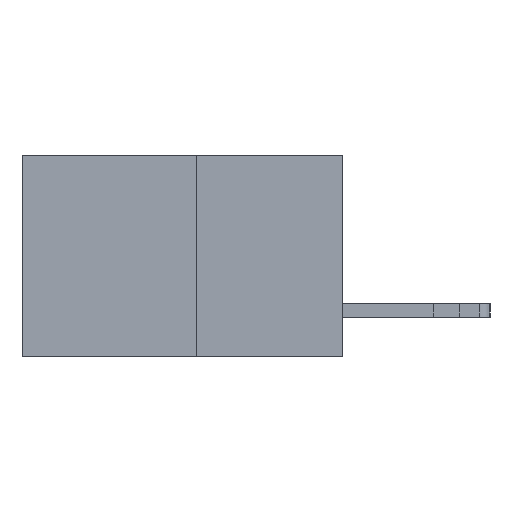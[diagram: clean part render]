
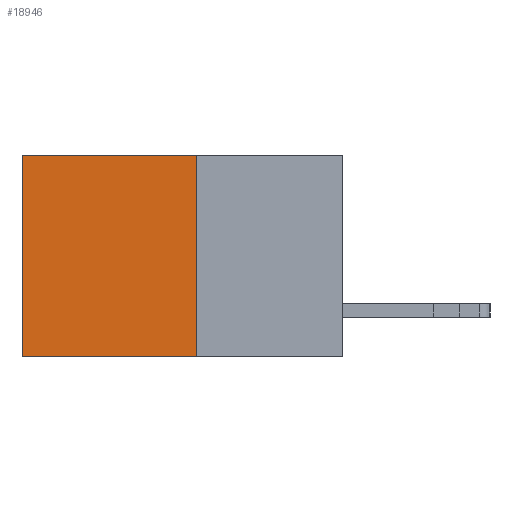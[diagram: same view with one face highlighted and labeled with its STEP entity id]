
A CAD part, left-side view. The second image highlights one B-rep face of the part: STEP entity #18946.
In plain terms, the highlighted planar face has unit normal (-1, 0, 0).
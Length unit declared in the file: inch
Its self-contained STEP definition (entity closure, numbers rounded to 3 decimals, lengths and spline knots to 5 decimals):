
#182 = VERTEX_POINT ( 'NONE', #16999 ) ;
#512 = CARTESIAN_POINT ( 'NONE',  ( 0.277, 0.59, -0.37 ) ) ;
#1148 = LINE ( 'NONE', #18157, #5114 ) ;
#2264 = DIRECTION ( 'NONE',  ( 0., 1., 0. ) ) ;
#2937 = EDGE_CURVE ( 'NONE', #14683, #4528, #1148, .T. ) ;
#3550 = ORIENTED_EDGE ( 'NONE', *, *, #5866, .T. ) ;
#3700 = CARTESIAN_POINT ( 'NONE',  ( 0.277, 0.27, -0.37 ) ) ;
#3926 = DIRECTION ( 'NONE',  ( 1., 0., 0. ) ) ;
#4033 = VECTOR ( 'NONE', #2264, 39.37008 ) ;
#4528 = VERTEX_POINT ( 'NONE', #512 ) ;
#5114 = VECTOR ( 'NONE', #18173, 39.37008 ) ;
#5172 = EDGE_CURVE ( 'NONE', #182, #11938, #16331, .T. ) ;
#5866 = EDGE_CURVE ( 'NONE', #182, #14683, #16510, .T. ) ;
#6033 = DIRECTION ( 'NONE',  ( 0., 0., -1. ) ) ;
#6759 = CARTESIAN_POINT ( 'NONE',  ( 0.277, 0.59, 0. ) ) ;
#6814 = EDGE_CURVE ( 'NONE', #11938, #4528, #11932, .T. ) ;
#7011 = EDGE_LOOP ( 'NONE', ( #18962, #16197, #15027, #3550 ) ) ;
#7658 = DIRECTION ( 'NONE',  ( 0., 1., 0. ) ) ;
#11932 = LINE ( 'NONE', #3700, #4033 ) ;
#11938 = VERTEX_POINT ( 'NONE', #19055 ) ;
#12143 = AXIS2_PLACEMENT_3D ( 'NONE', #12838, #3926, #14366 ) ;
#12436 = VECTOR ( 'NONE', #7658, 39.37008 ) ;
#12838 = CARTESIAN_POINT ( 'NONE',  ( 0.277, 0.27, -0.37 ) ) ;
#13456 = CARTESIAN_POINT ( 'NONE',  ( 0.277, 0.27, -0.37 ) ) ;
#13560 = CARTESIAN_POINT ( 'NONE',  ( 0.277, 0.27, 0. ) ) ;
#14366 = DIRECTION ( 'NONE',  ( 0., 0., -1. ) ) ;
#14683 = VERTEX_POINT ( 'NONE', #6759 ) ;
#15027 = ORIENTED_EDGE ( 'NONE', *, *, #5172, .F. ) ;
#15356 = VECTOR ( 'NONE', #6033, 39.37008 ) ;
#15606 = FACE_OUTER_BOUND ( 'NONE', #7011, .T. ) ;
#16197 = ORIENTED_EDGE ( 'NONE', *, *, #6814, .F. ) ;
#16331 = LINE ( 'NONE', #13456, #15356 ) ;
#16510 = LINE ( 'NONE', #13560, #12436 ) ;
#16999 = CARTESIAN_POINT ( 'NONE',  ( 0.277, 0.27, 0. ) ) ;
#17396 = PLANE ( 'NONE',  #12143 ) ;
#18157 = CARTESIAN_POINT ( 'NONE',  ( 0.277, 0.59, -0.37 ) ) ;
#18173 = DIRECTION ( 'NONE',  ( 0., 0., -1. ) ) ;
#18946 = ADVANCED_FACE ( 'NONE', ( #15606 ), #17396, .F. ) ;
#18962 = ORIENTED_EDGE ( 'NONE', *, *, #2937, .T. ) ;
#19055 = CARTESIAN_POINT ( 'NONE',  ( 0.277, 0.27, -0.37 ) ) ;
